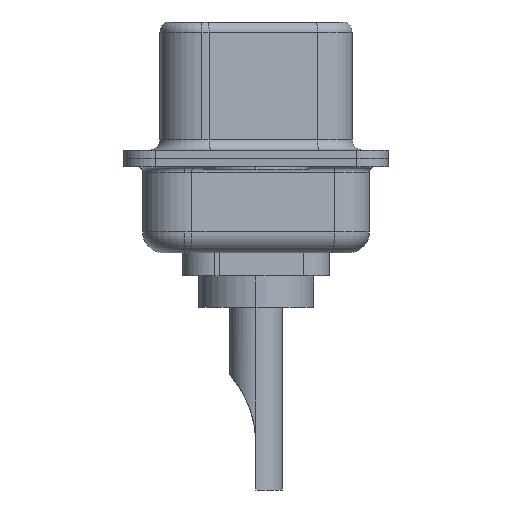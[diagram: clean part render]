
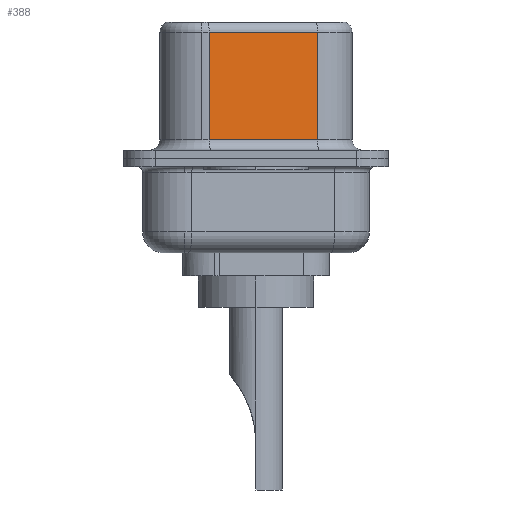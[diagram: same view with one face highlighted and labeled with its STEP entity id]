
A CAD part, left-side view. The second image highlights one B-rep face of the part: STEP entity #388.
In plain terms, the highlighted planar face has unit normal (-0.985, -0.174, 0).
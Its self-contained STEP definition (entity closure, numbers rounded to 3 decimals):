
#91 = ORIENTED_EDGE ( 'NONE', *, *, #13926, .T. ) ;
#296 = AXIS2_PLACEMENT_3D ( 'NONE', #7082, #9456, #5233 ) ;
#388 = ADVANCED_FACE ( 'NONE', ( #1563 ), #12233, .F. ) ;
#602 = EDGE_LOOP ( 'NONE', ( #10934, #1531, #91, #8984 ) ) ;
#656 = VECTOR ( 'NONE', #3679, 1000. ) ;
#1104 = CARTESIAN_POINT ( 'NONE',  ( 4.565, -2.927, 6.52 ) ) ;
#1531 = ORIENTED_EDGE ( 'NONE', *, *, #9984, .T. ) ;
#1563 = FACE_OUTER_BOUND ( 'NONE', #602, .T. ) ;
#1855 = DIRECTION ( 'NONE',  ( 0.174, -0.985, 0. ) ) ;
#1976 = CARTESIAN_POINT ( 'NONE',  ( 3.655, 2.233, 6.02 ) ) ;
#2959 = EDGE_CURVE ( 'NONE', #12108, #10702, #4641, .T. ) ;
#3679 = DIRECTION ( 'NONE',  ( -0.174, 0.985, 0. ) ) ;
#4297 = VECTOR ( 'NONE', #1855, 1000. ) ;
#4641 = LINE ( 'NONE', #9398, #4297 ) ;
#5233 = DIRECTION ( 'NONE',  ( -0.174, 0.985, 0. ) ) ;
#6492 = LINE ( 'NONE', #6919, #656 ) ;
#6504 = CARTESIAN_POINT ( 'NONE',  ( 3.655, 2.233, 6.52 ) ) ;
#6919 = CARTESIAN_POINT ( 'NONE',  ( 4.565, -2.927, 6.02 ) ) ;
#7082 = CARTESIAN_POINT ( 'NONE',  ( 4.565, -2.927, 6.52 ) ) ;
#7600 = DIRECTION ( 'NONE',  ( 0., 0., -1. ) ) ;
#8113 = VECTOR ( 'NONE', #7600, 1000. ) ;
#8984 = ORIENTED_EDGE ( 'NONE', *, *, #2959, .T. ) ;
#9398 = CARTESIAN_POINT ( 'NONE',  ( 4.565, -2.927, 0.9 ) ) ;
#9456 = DIRECTION ( 'NONE',  ( 0.985, 0.174, 0. ) ) ;
#9773 = DIRECTION ( 'NONE',  ( 0., 0., -1. ) ) ;
#9984 = EDGE_CURVE ( 'NONE', #12178, #13540, #6492, .T. ) ;
#10702 = VERTEX_POINT ( 'NONE', #11430 ) ;
#10934 = ORIENTED_EDGE ( 'NONE', *, *, #11254, .F. ) ;
#11021 = LINE ( 'NONE', #1104, #8113 ) ;
#11123 = VECTOR ( 'NONE', #9773, 1000. ) ;
#11254 = EDGE_CURVE ( 'NONE', #12178, #10702, #11021, .T. ) ;
#11430 = CARTESIAN_POINT ( 'NONE',  ( 4.565, -2.927, 0.9 ) ) ;
#12108 = VERTEX_POINT ( 'NONE', #13444 ) ;
#12178 = VERTEX_POINT ( 'NONE', #12527 ) ;
#12233 = PLANE ( 'NONE',  #296 ) ;
#12527 = CARTESIAN_POINT ( 'NONE',  ( 4.565, -2.927, 6.02 ) ) ;
#13444 = CARTESIAN_POINT ( 'NONE',  ( 3.655, 2.233, 0.9 ) ) ;
#13540 = VERTEX_POINT ( 'NONE', #1976 ) ;
#13926 = EDGE_CURVE ( 'NONE', #13540, #12108, #14020, .T. ) ;
#14020 = LINE ( 'NONE', #6504, #11123 ) ;
